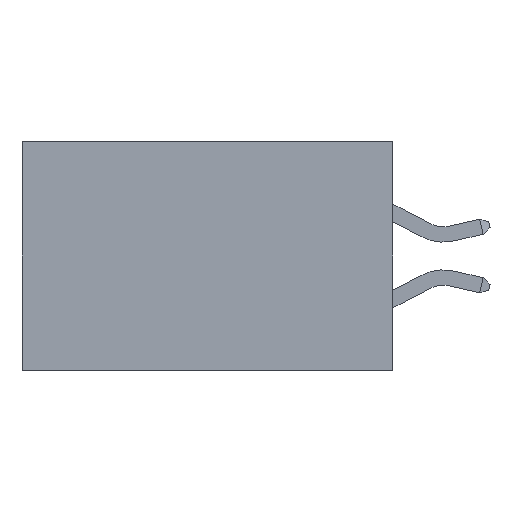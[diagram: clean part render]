
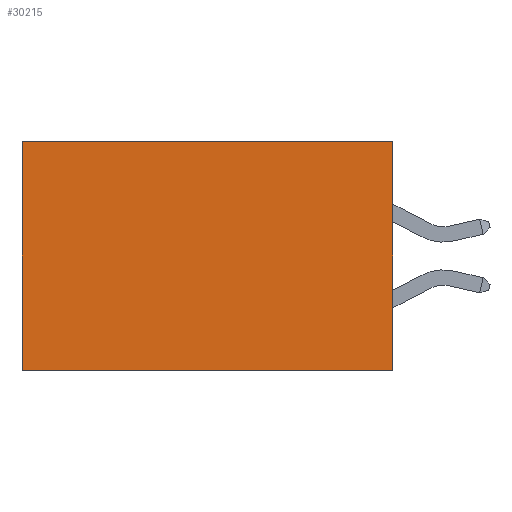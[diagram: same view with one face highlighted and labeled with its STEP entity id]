
A CAD part, left-side view. The second image highlights one B-rep face of the part: STEP entity #30215.
In plain terms, the highlighted planar face has unit normal (-1, 0, 0).
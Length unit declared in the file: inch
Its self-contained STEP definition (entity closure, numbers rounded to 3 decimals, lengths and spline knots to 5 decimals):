
#352 = EDGE_LOOP ( 'NONE', ( #16025, #27300, #16737, #22778 ) ) ;
#2976 = EDGE_CURVE ( 'NONE', #19833, #40150, #33287, .T. ) ;
#3298 = CARTESIAN_POINT ( 'NONE',  ( 0.2875, 0.6, -0.37 ) ) ;
#4114 = DIRECTION ( 'NONE',  ( 1., 0., 0. ) ) ;
#5111 = CARTESIAN_POINT ( 'NONE',  ( 0.2875, 0., -0.37 ) ) ;
#5845 = AXIS2_PLACEMENT_3D ( 'NONE', #30143, #4114, #26985 ) ;
#5931 = DIRECTION ( 'NONE',  ( 0., 0., -1. ) ) ;
#6884 = DIRECTION ( 'NONE',  ( 0., 0., -1. ) ) ;
#9354 = VECTOR ( 'NONE', #38376, 39.37008 ) ;
#10483 = FACE_OUTER_BOUND ( 'NONE', #352, .T. ) ;
#14163 = EDGE_CURVE ( 'NONE', #19833, #19686, #35328, .T. ) ;
#14430 = CARTESIAN_POINT ( 'NONE',  ( 0.2875, 0., 0. ) ) ;
#16025 = ORIENTED_EDGE ( 'NONE', *, *, #26196, .T. ) ;
#16737 = ORIENTED_EDGE ( 'NONE', *, *, #2976, .F. ) ;
#18965 = CARTESIAN_POINT ( 'NONE',  ( 0.2875, 0.6, 0. ) ) ;
#19686 = VERTEX_POINT ( 'NONE', #31045 ) ;
#19833 = VERTEX_POINT ( 'NONE', #38166 ) ;
#22778 = ORIENTED_EDGE ( 'NONE', *, *, #14163, .T. ) ;
#23743 = PLANE ( 'NONE',  #5845 ) ;
#25961 = VECTOR ( 'NONE', #37704, 39.37008 ) ;
#26196 = EDGE_CURVE ( 'NONE', #19686, #34097, #39762, .T. ) ;
#26985 = DIRECTION ( 'NONE',  ( 0., 0., -1. ) ) ;
#27300 = ORIENTED_EDGE ( 'NONE', *, *, #34473, .F. ) ;
#30143 = CARTESIAN_POINT ( 'NONE',  ( 0.2875, 0., 0. ) ) ;
#30215 = ADVANCED_FACE ( 'NONE', ( #10483 ), #23743, .F. ) ;
#31045 = CARTESIAN_POINT ( 'NONE',  ( 0.2875, 0.6, 0. ) ) ;
#33287 = LINE ( 'NONE', #14430, #38752 ) ;
#33583 = LINE ( 'NONE', #5111, #25961 ) ;
#34097 = VERTEX_POINT ( 'NONE', #3298 ) ;
#34473 = EDGE_CURVE ( 'NONE', #40150, #34097, #33583, .T. ) ;
#35328 = LINE ( 'NONE', #41592, #9354 ) ;
#35950 = CARTESIAN_POINT ( 'NONE',  ( 0.2875, 0., -0.37 ) ) ;
#37704 = DIRECTION ( 'NONE',  ( 0., 1., 0. ) ) ;
#38166 = CARTESIAN_POINT ( 'NONE',  ( 0.2875, 0., 0. ) ) ;
#38376 = DIRECTION ( 'NONE',  ( 0., 1., 0. ) ) ;
#38733 = VECTOR ( 'NONE', #5931, 39.37008 ) ;
#38752 = VECTOR ( 'NONE', #6884, 39.37008 ) ;
#39762 = LINE ( 'NONE', #18965, #38733 ) ;
#40150 = VERTEX_POINT ( 'NONE', #35950 ) ;
#41592 = CARTESIAN_POINT ( 'NONE',  ( 0.2875, 0., 0. ) ) ;
